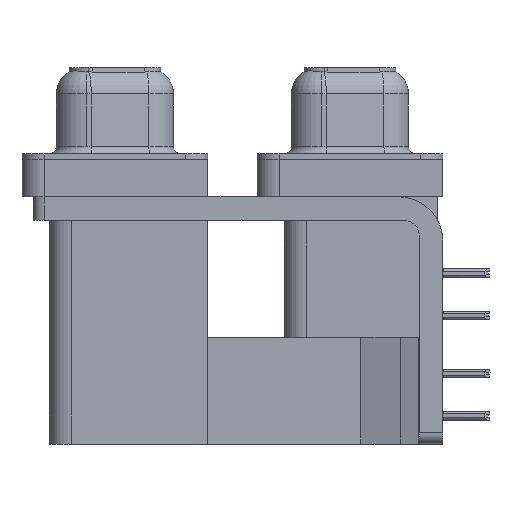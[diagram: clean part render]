
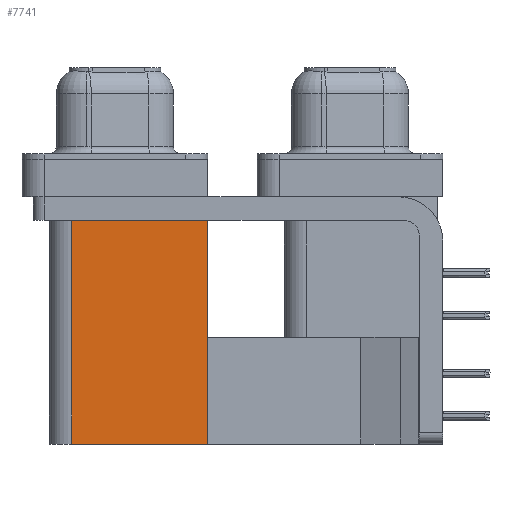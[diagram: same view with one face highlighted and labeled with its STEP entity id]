
A CAD part, left-side view. The second image highlights one B-rep face of the part: STEP entity #7741.
In plain terms, the highlighted planar face has unit normal (-1, 0, 0).
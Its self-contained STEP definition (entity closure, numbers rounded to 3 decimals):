
#305 = DIRECTION ( 'NONE',  ( 0., 0., 1. ) ) ;
#369 = DIRECTION ( 'NONE',  ( 0., 1., 0. ) ) ;
#667 = VERTEX_POINT ( 'NONE', #9809 ) ;
#2210 = ORIENTED_EDGE ( 'NONE', *, *, #5524, .F. ) ;
#2314 = CARTESIAN_POINT ( 'NONE',  ( 3.79, 18.8, -2.5 ) ) ;
#2573 = DIRECTION ( 'NONE',  ( 0., 1., 0. ) ) ;
#2935 = CARTESIAN_POINT ( 'NONE',  ( 3.79, 9.6, -19.2 ) ) ;
#5524 = EDGE_CURVE ( 'NONE', #667, #14535, #14296, .T. ) ;
#5650 = CARTESIAN_POINT ( 'NONE',  ( 3.79, 9.6, -19.2 ) ) ;
#6836 = AXIS2_PLACEMENT_3D ( 'NONE', #12221, #19211, #35543 ) ;
#7741 = ADVANCED_FACE ( 'NONE', ( #29175 ), #22611, .F. ) ;
#9809 = CARTESIAN_POINT ( 'NONE',  ( 3.79, 18.8, -19.2 ) ) ;
#10309 = EDGE_CURVE ( 'NONE', #36091, #667, #36273, .T. ) ;
#11075 = VECTOR ( 'NONE', #2573, 1000. ) ;
#11831 = DIRECTION ( 'NONE',  ( 0., 0., 1. ) ) ;
#12221 = CARTESIAN_POINT ( 'NONE',  ( 3.79, 9.6, -19.2 ) ) ;
#12892 = EDGE_CURVE ( 'NONE', #22940, #14535, #24890, .T. ) ;
#13499 = CARTESIAN_POINT ( 'NONE',  ( 3.79, 18.8, -19.2 ) ) ;
#14296 = LINE ( 'NONE', #13499, #20205 ) ;
#14535 = VERTEX_POINT ( 'NONE', #2314 ) ;
#18139 = ORIENTED_EDGE ( 'NONE', *, *, #20431, .T. ) ;
#18650 = ORIENTED_EDGE ( 'NONE', *, *, #10309, .F. ) ;
#19211 = DIRECTION ( 'NONE',  ( 1., 0., 0. ) ) ;
#20205 = VECTOR ( 'NONE', #305, 1000. ) ;
#20431 = EDGE_CURVE ( 'NONE', #36091, #22940, #31366, .T. ) ;
#20947 = ORIENTED_EDGE ( 'NONE', *, *, #12892, .T. ) ;
#22611 = PLANE ( 'NONE',  #6836 ) ;
#22940 = VERTEX_POINT ( 'NONE', #24332 ) ;
#24048 = EDGE_LOOP ( 'NONE', ( #20947, #2210, #18650, #18139 ) ) ;
#24332 = CARTESIAN_POINT ( 'NONE',  ( 3.79, 9.6, -2.5 ) ) ;
#24890 = LINE ( 'NONE', #34034, #11075 ) ;
#25039 = VECTOR ( 'NONE', #11831, 1000. ) ;
#29175 = FACE_OUTER_BOUND ( 'NONE', #24048, .T. ) ;
#31366 = LINE ( 'NONE', #5650, #25039 ) ;
#34034 = CARTESIAN_POINT ( 'NONE',  ( 3.79, 9.6, -2.5 ) ) ;
#35543 = DIRECTION ( 'NONE',  ( 0., 1., 0. ) ) ;
#36091 = VERTEX_POINT ( 'NONE', #2935 ) ;
#36273 = LINE ( 'NONE', #39050, #40065 ) ;
#39050 = CARTESIAN_POINT ( 'NONE',  ( 3.79, 9.6, -19.2 ) ) ;
#40065 = VECTOR ( 'NONE', #369, 1000. ) ;
